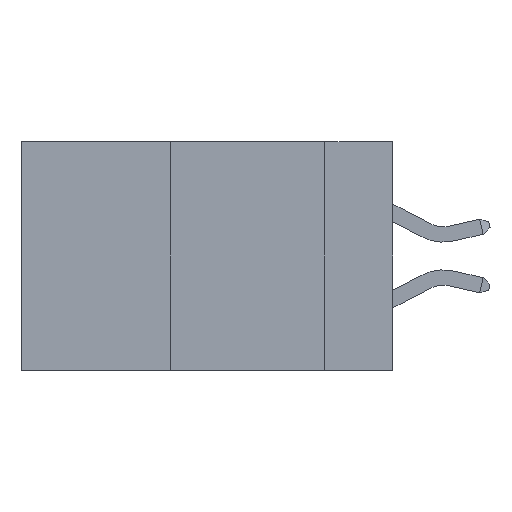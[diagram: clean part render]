
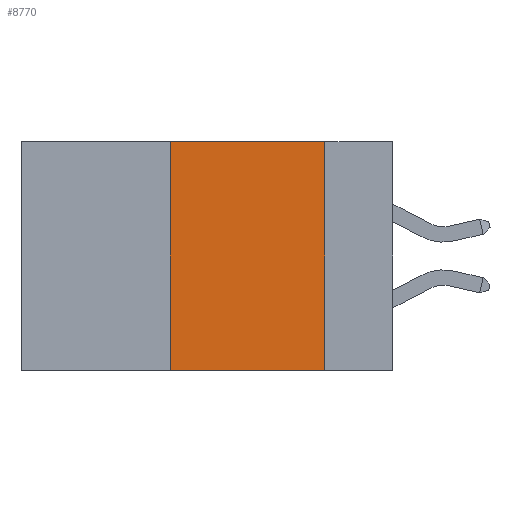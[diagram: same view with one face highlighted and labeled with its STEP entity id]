
A CAD part, left-side view. The second image highlights one B-rep face of the part: STEP entity #8770.
In plain terms, the highlighted planar face has unit normal (-1, 0, 0).
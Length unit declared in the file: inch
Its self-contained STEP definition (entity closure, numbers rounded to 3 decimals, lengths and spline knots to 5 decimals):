
#769 = DIRECTION ( 'NONE',  ( 0., -1., 0. ) ) ;
#915 = DIRECTION ( 'NONE',  ( 1., 0., 0. ) ) ;
#1223 = VERTEX_POINT ( 'NONE', #21691 ) ;
#2331 = EDGE_LOOP ( 'NONE', ( #15782, #21316, #11843, #16959 ) ) ;
#2408 = CARTESIAN_POINT ( 'NONE',  ( 0., 0.36, 0. ) ) ;
#3386 = LINE ( 'NONE', #6206, #8041 ) ;
#4265 = VERTEX_POINT ( 'NONE', #20826 ) ;
#4348 = VECTOR ( 'NONE', #769, 39.37008 ) ;
#6206 = CARTESIAN_POINT ( 'NONE',  ( 0., 0.36, 0. ) ) ;
#6235 = LINE ( 'NONE', #8857, #20375 ) ;
#7404 = DIRECTION ( 'NONE',  ( 0., 0., -1. ) ) ;
#8041 = VECTOR ( 'NONE', #14074, 39.37008 ) ;
#8770 = ADVANCED_FACE ( 'NONE', ( #23203 ), #16511, .F. ) ;
#8857 = CARTESIAN_POINT ( 'NONE',  ( 0., 0.6, -0.37 ) ) ;
#9229 = EDGE_CURVE ( 'NONE', #1223, #22657, #3386, .T. ) ;
#11296 = LINE ( 'NONE', #18896, #21362 ) ;
#11843 = ORIENTED_EDGE ( 'NONE', *, *, #9229, .F. ) ;
#12795 = DIRECTION ( 'NONE',  ( 0., -1., 0. ) ) ;
#13101 = AXIS2_PLACEMENT_3D ( 'NONE', #20269, #915, #14695 ) ;
#14074 = DIRECTION ( 'NONE',  ( 0., 0., 1. ) ) ;
#14543 = CARTESIAN_POINT ( 'NONE',  ( 0., 0.6, 0. ) ) ;
#14695 = DIRECTION ( 'NONE',  ( 0., 0., -1. ) ) ;
#15740 = EDGE_CURVE ( 'NONE', #1223, #4265, #6235, .T. ) ;
#15782 = ORIENTED_EDGE ( 'NONE', *, *, #21200, .F. ) ;
#16209 = EDGE_CURVE ( 'NONE', #22657, #21728, #24055, .T. ) ;
#16511 = PLANE ( 'NONE',  #13101 ) ;
#16959 = ORIENTED_EDGE ( 'NONE', *, *, #15740, .T. ) ;
#18628 = CARTESIAN_POINT ( 'NONE',  ( 0., 0.11, 0. ) ) ;
#18896 = CARTESIAN_POINT ( 'NONE',  ( 0., 0.11, 0. ) ) ;
#20269 = CARTESIAN_POINT ( 'NONE',  ( 0., 0.6, 0. ) ) ;
#20375 = VECTOR ( 'NONE', #12795, 39.37008 ) ;
#20826 = CARTESIAN_POINT ( 'NONE',  ( 0., 0.11, -0.37 ) ) ;
#21200 = EDGE_CURVE ( 'NONE', #21728, #4265, #11296, .T. ) ;
#21316 = ORIENTED_EDGE ( 'NONE', *, *, #16209, .F. ) ;
#21362 = VECTOR ( 'NONE', #7404, 39.37008 ) ;
#21691 = CARTESIAN_POINT ( 'NONE',  ( 0., 0.36, -0.37 ) ) ;
#21728 = VERTEX_POINT ( 'NONE', #18628 ) ;
#22657 = VERTEX_POINT ( 'NONE', #2408 ) ;
#23203 = FACE_OUTER_BOUND ( 'NONE', #2331, .T. ) ;
#24055 = LINE ( 'NONE', #14543, #4348 ) ;
